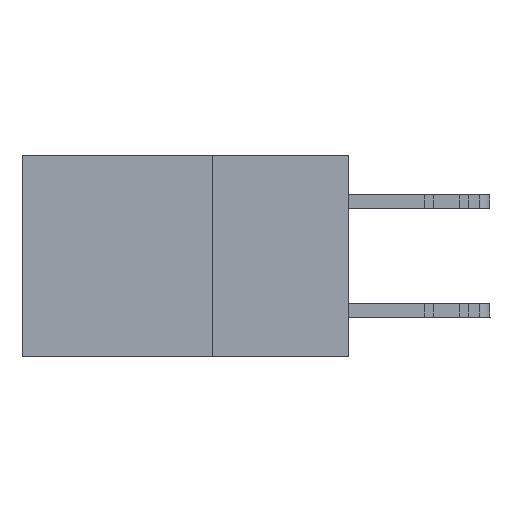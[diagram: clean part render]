
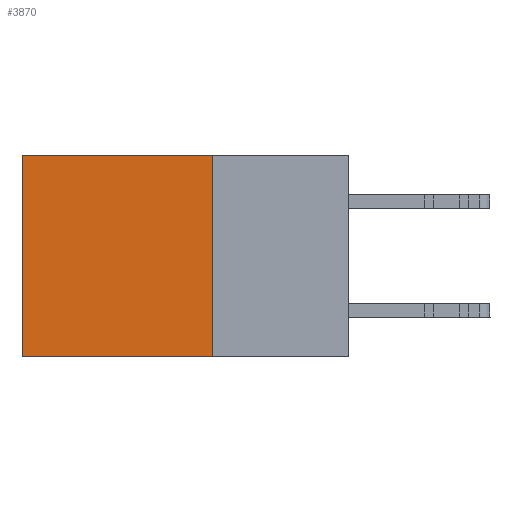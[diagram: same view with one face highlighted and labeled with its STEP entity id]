
A CAD part, left-side view. The second image highlights one B-rep face of the part: STEP entity #3870.
In plain terms, the highlighted planar face has unit normal (-1, 0, 0).
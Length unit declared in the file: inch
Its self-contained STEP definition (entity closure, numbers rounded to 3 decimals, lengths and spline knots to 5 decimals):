
#2281 = LINE ( 'NONE', #19102, #9077 ) ;
#3765 = DIRECTION ( 'NONE',  ( 0., 1., 0. ) ) ;
#3870 = ADVANCED_FACE ( 'NONE', ( #31079 ), #17484, .F. ) ;
#4724 = DIRECTION ( 'NONE',  ( 1., 0., 0. ) ) ;
#5282 = CARTESIAN_POINT ( 'NONE',  ( 0.298, 0.6, 0. ) ) ;
#5509 = EDGE_LOOP ( 'NONE', ( #6221, #26273, #20354, #26425 ) ) ;
#5991 = EDGE_CURVE ( 'NONE', #30517, #12621, #19032, .T. ) ;
#6221 = ORIENTED_EDGE ( 'NONE', *, *, #5991, .T. ) ;
#8256 = CARTESIAN_POINT ( 'NONE',  ( 0.298, 0.25, 0. ) ) ;
#9077 = VECTOR ( 'NONE', #3765, 39.37008 ) ;
#10826 = EDGE_CURVE ( 'NONE', #21528, #15694, #26742, .T. ) ;
#11541 = VECTOR ( 'NONE', #26248, 39.37008 ) ;
#11723 = CARTESIAN_POINT ( 'NONE',  ( 0.298, 0.6, 0. ) ) ;
#12621 = VERTEX_POINT ( 'NONE', #30830 ) ;
#13169 = CARTESIAN_POINT ( 'NONE',  ( 0.298, 0.25, 0. ) ) ;
#15694 = VERTEX_POINT ( 'NONE', #26247 ) ;
#16409 = LINE ( 'NONE', #25320, #30003 ) ;
#17484 = PLANE ( 'NONE',  #25042 ) ;
#19032 = LINE ( 'NONE', #5282, #31780 ) ;
#19102 = CARTESIAN_POINT ( 'NONE',  ( 0.298, 0.25, 0. ) ) ;
#20058 = CARTESIAN_POINT ( 'NONE',  ( 0.298, 0.25, 0. ) ) ;
#20354 = ORIENTED_EDGE ( 'NONE', *, *, #10826, .F. ) ;
#21528 = VERTEX_POINT ( 'NONE', #13169 ) ;
#22623 = DIRECTION ( 'NONE',  ( 0., 0., -1. ) ) ;
#23178 = DIRECTION ( 'NONE',  ( 0., 0., -1. ) ) ;
#23996 = EDGE_CURVE ( 'NONE', #21528, #30517, #2281, .T. ) ;
#25042 = AXIS2_PLACEMENT_3D ( 'NONE', #20058, #4724, #22623 ) ;
#25320 = CARTESIAN_POINT ( 'NONE',  ( 0.298, 0.25, -0.37 ) ) ;
#26247 = CARTESIAN_POINT ( 'NONE',  ( 0.298, 0.25, -0.37 ) ) ;
#26248 = DIRECTION ( 'NONE',  ( 0., 0., -1. ) ) ;
#26273 = ORIENTED_EDGE ( 'NONE', *, *, #30752, .F. ) ;
#26425 = ORIENTED_EDGE ( 'NONE', *, *, #23996, .T. ) ;
#26742 = LINE ( 'NONE', #8256, #11541 ) ;
#30003 = VECTOR ( 'NONE', #32999, 39.37008 ) ;
#30517 = VERTEX_POINT ( 'NONE', #11723 ) ;
#30752 = EDGE_CURVE ( 'NONE', #15694, #12621, #16409, .T. ) ;
#30830 = CARTESIAN_POINT ( 'NONE',  ( 0.298, 0.6, -0.37 ) ) ;
#31079 = FACE_OUTER_BOUND ( 'NONE', #5509, .T. ) ;
#31780 = VECTOR ( 'NONE', #23178, 39.37008 ) ;
#32999 = DIRECTION ( 'NONE',  ( 0., 1., 0. ) ) ;
